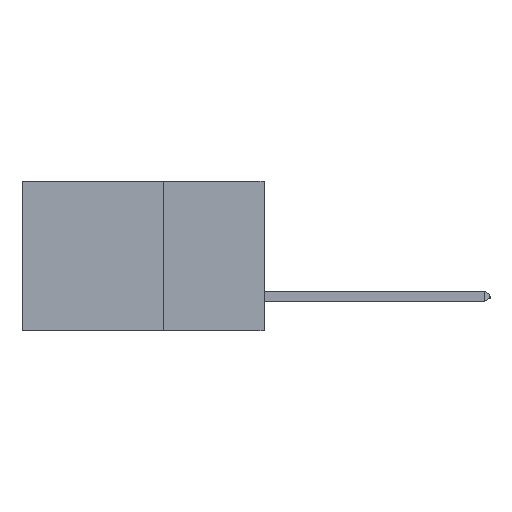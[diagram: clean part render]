
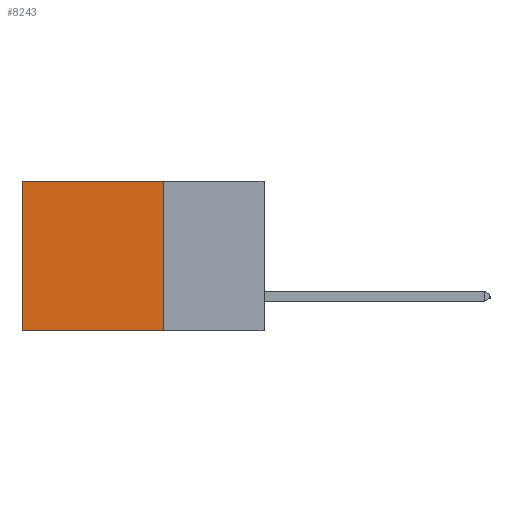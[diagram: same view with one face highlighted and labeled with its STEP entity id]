
A CAD part, left-side view. The second image highlights one B-rep face of the part: STEP entity #8243.
In plain terms, the highlighted planar face has unit normal (-1, 0, 0).
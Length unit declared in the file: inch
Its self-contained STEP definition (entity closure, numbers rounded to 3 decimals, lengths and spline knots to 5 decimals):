
#143 = VECTOR ( 'NONE', #12884, 39.37008 ) ;
#861 = CARTESIAN_POINT ( 'NONE',  ( 0.298, 0.25, -0.37 ) ) ;
#933 = VECTOR ( 'NONE', #11970, 39.37008 ) ;
#1068 = VERTEX_POINT ( 'NONE', #11786 ) ;
#1283 = AXIS2_PLACEMENT_3D ( 'NONE', #8715, #1594, #9898 ) ;
#1594 = DIRECTION ( 'NONE',  ( 1., 0., 0. ) ) ;
#2062 = VERTEX_POINT ( 'NONE', #861 ) ;
#2396 = EDGE_LOOP ( 'NONE', ( #8215, #6328, #14848, #11013 ) ) ;
#2497 = VERTEX_POINT ( 'NONE', #6212 ) ;
#3310 = VECTOR ( 'NONE', #10653, 39.37008 ) ;
#3488 = LINE ( 'NONE', #9227, #6656 ) ;
#3693 = LINE ( 'NONE', #5703, #3310 ) ;
#3996 = EDGE_CURVE ( 'NONE', #1068, #2497, #3693, .T. ) ;
#4834 = EDGE_CURVE ( 'NONE', #2062, #8418, #12718, .T. ) ;
#5703 = CARTESIAN_POINT ( 'NONE',  ( 0.298, 0.25, 0. ) ) ;
#6212 = CARTESIAN_POINT ( 'NONE',  ( 0.298, 0.6, 0. ) ) ;
#6328 = ORIENTED_EDGE ( 'NONE', *, *, #4834, .F. ) ;
#6656 = VECTOR ( 'NONE', #6883, 39.37008 ) ;
#6883 = DIRECTION ( 'NONE',  ( 0., 0., -1. ) ) ;
#8129 = EDGE_CURVE ( 'NONE', #1068, #2062, #10395, .T. ) ;
#8215 = ORIENTED_EDGE ( 'NONE', *, *, #10115, .T. ) ;
#8243 = ADVANCED_FACE ( 'NONE', ( #14366 ), #14500, .F. ) ;
#8418 = VERTEX_POINT ( 'NONE', #11356 ) ;
#8715 = CARTESIAN_POINT ( 'NONE',  ( 0.298, 0.25, 0. ) ) ;
#9227 = CARTESIAN_POINT ( 'NONE',  ( 0.298, 0.6, 0. ) ) ;
#9898 = DIRECTION ( 'NONE',  ( 0., 0., -1. ) ) ;
#10115 = EDGE_CURVE ( 'NONE', #2497, #8418, #3488, .T. ) ;
#10395 = LINE ( 'NONE', #13137, #933 ) ;
#10563 = CARTESIAN_POINT ( 'NONE',  ( 0.298, 0.25, -0.37 ) ) ;
#10653 = DIRECTION ( 'NONE',  ( 0., 1., 0. ) ) ;
#11013 = ORIENTED_EDGE ( 'NONE', *, *, #3996, .T. ) ;
#11356 = CARTESIAN_POINT ( 'NONE',  ( 0.298, 0.6, -0.37 ) ) ;
#11786 = CARTESIAN_POINT ( 'NONE',  ( 0.298, 0.25, 0. ) ) ;
#11970 = DIRECTION ( 'NONE',  ( 0., 0., -1. ) ) ;
#12718 = LINE ( 'NONE', #10563, #143 ) ;
#12884 = DIRECTION ( 'NONE',  ( 0., 1., 0. ) ) ;
#13137 = CARTESIAN_POINT ( 'NONE',  ( 0.298, 0.25, 0. ) ) ;
#14366 = FACE_OUTER_BOUND ( 'NONE', #2396, .T. ) ;
#14500 = PLANE ( 'NONE',  #1283 ) ;
#14848 = ORIENTED_EDGE ( 'NONE', *, *, #8129, .F. ) ;
